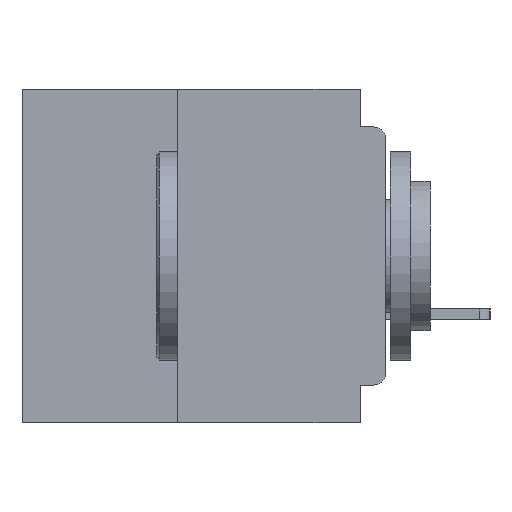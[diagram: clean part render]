
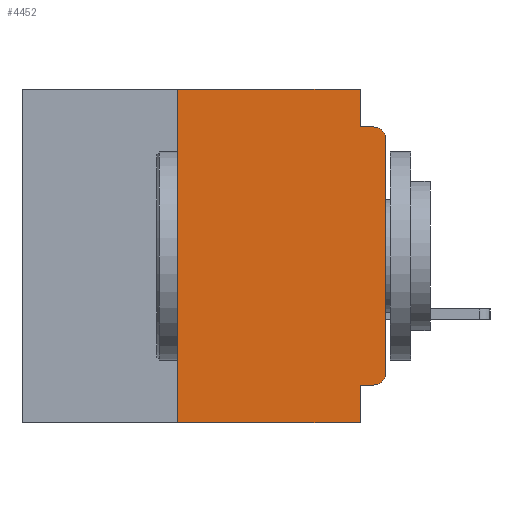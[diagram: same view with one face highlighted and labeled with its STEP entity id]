
A CAD part, left-side view. The second image highlights one B-rep face of the part: STEP entity #4452.
In plain terms, the highlighted planar face has unit normal (-1, 0, 0).
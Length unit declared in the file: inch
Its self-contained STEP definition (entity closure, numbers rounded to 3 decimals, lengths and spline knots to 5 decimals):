
#224 = LINE ( 'NONE', #22350, #27038 ) ;
#269 = EDGE_CURVE ( 'NONE', #44445, #28479, #2265, .T. ) ;
#1649 = EDGE_CURVE ( 'NONE', #26381, #44512, #7713, .T. ) ;
#1786 = AXIS2_PLACEMENT_3D ( 'NONE', #3555, #2990, #2940 ) ;
#1820 = VERTEX_POINT ( 'NONE', #19392 ) ;
#2265 = LINE ( 'NONE', #32004, #29104 ) ;
#2416 = VERTEX_POINT ( 'NONE', #4908 ) ;
#2940 = DIRECTION ( 'NONE',  ( 0., 0., -1. ) ) ;
#2990 = DIRECTION ( 'NONE',  ( 1., 0., 0. ) ) ;
#3138 = PLANE ( 'NONE',  #1786 ) ;
#3555 = CARTESIAN_POINT ( 'NONE',  ( 0., 0.437, 0. ) ) ;
#4447 = CIRCLE ( 'NONE', #4671, 0.015 ) ;
#4452 = ADVANCED_FACE ( 'NONE', ( #10829 ), #3138, .F. ) ;
#4671 = AXIS2_PLACEMENT_3D ( 'NONE', #34723, #13765, #38203 ) ;
#4908 = CARTESIAN_POINT ( 'NONE',  ( 0., 0.031, -0.045 ) ) ;
#4934 = VERTEX_POINT ( 'NONE', #20865 ) ;
#5201 = CIRCLE ( 'NONE', #21143, 0.015 ) ;
#5865 = LINE ( 'NONE', #12156, #14056 ) ;
#7415 = CARTESIAN_POINT ( 'NONE',  ( 0., 0.437, 0. ) ) ;
#7713 = LINE ( 'NONE', #23816, #26300 ) ;
#7797 = ORIENTED_EDGE ( 'NONE', *, *, #37757, .T. ) ;
#8063 = CARTESIAN_POINT ( 'NONE',  ( 0., 0.015, -0.06 ) ) ;
#8681 = ORIENTED_EDGE ( 'NONE', *, *, #1649, .F. ) ;
#10325 = CARTESIAN_POINT ( 'NONE',  ( 0., 0.031, 0. ) ) ;
#10829 = FACE_OUTER_BOUND ( 'NONE', #17352, .T. ) ;
#10909 = DIRECTION ( 'NONE',  ( 0., -1., 0. ) ) ;
#10977 = CARTESIAN_POINT ( 'NONE',  ( 0., 0., -0.045 ) ) ;
#11052 = EDGE_CURVE ( 'NONE', #34389, #2416, #5865, .T. ) ;
#11077 = ORIENTED_EDGE ( 'NONE', *, *, #31630, .T. ) ;
#11319 = ORIENTED_EDGE ( 'NONE', *, *, #22314, .T. ) ;
#11426 = CARTESIAN_POINT ( 'NONE',  ( 0., 0.015, -0.045 ) ) ;
#11463 = EDGE_CURVE ( 'NONE', #44512, #34389, #32624, .T. ) ;
#11566 = DIRECTION ( 'NONE',  ( 0., 0., -1. ) ) ;
#11826 = VECTOR ( 'NONE', #21428, 39.37008 ) ;
#12156 = CARTESIAN_POINT ( 'NONE',  ( 0., 0.031, 0. ) ) ;
#13763 = CARTESIAN_POINT ( 'NONE',  ( 0., 0.437, -0.4 ) ) ;
#13765 = DIRECTION ( 'NONE',  ( -1., 0., 0. ) ) ;
#14056 = VECTOR ( 'NONE', #40115, 39.37008 ) ;
#14590 = ORIENTED_EDGE ( 'NONE', *, *, #269, .F. ) ;
#16676 = EDGE_CURVE ( 'NONE', #2416, #35874, #30441, .T. ) ;
#17352 = EDGE_LOOP ( 'NONE', ( #7797, #11077, #20980, #42593, #22431, #8681, #31587, #39763, #14590, #11319 ) ) ;
#17910 = CARTESIAN_POINT ( 'NONE',  ( 0., 0.25, 0. ) ) ;
#19392 = CARTESIAN_POINT ( 'NONE',  ( 0., 0., -0.06 ) ) ;
#20865 = CARTESIAN_POINT ( 'NONE',  ( 0., 0.031, -0.4 ) ) ;
#20980 = ORIENTED_EDGE ( 'NONE', *, *, #16676, .F. ) ;
#21023 = CARTESIAN_POINT ( 'NONE',  ( 0., 0.015, -0.355 ) ) ;
#21143 = AXIS2_PLACEMENT_3D ( 'NONE', #8063, #32520, #11566 ) ;
#21428 = DIRECTION ( 'NONE',  ( 0., -1., 0. ) ) ;
#22265 = CARTESIAN_POINT ( 'NONE',  ( 0., 0.25, -0.4 ) ) ;
#22314 = EDGE_CURVE ( 'NONE', #44445, #32727, #4447, .T. ) ;
#22350 = CARTESIAN_POINT ( 'NONE',  ( 0., 0.031, -0.4 ) ) ;
#22431 = ORIENTED_EDGE ( 'NONE', *, *, #11463, .F. ) ;
#23705 = DIRECTION ( 'NONE',  ( 0., 0., 1. ) ) ;
#23816 = CARTESIAN_POINT ( 'NONE',  ( 0., 0.25, -0.4 ) ) ;
#26267 = CARTESIAN_POINT ( 'NONE',  ( 0., 0., 0. ) ) ;
#26300 = VECTOR ( 'NONE', #23705, 39.37008 ) ;
#26381 = VERTEX_POINT ( 'NONE', #22265 ) ;
#27038 = VECTOR ( 'NONE', #36353, 39.37008 ) ;
#28479 = VERTEX_POINT ( 'NONE', #34194 ) ;
#29104 = VECTOR ( 'NONE', #32100, 39.37008 ) ;
#29774 = DIRECTION ( 'NONE',  ( 0., 0., 1. ) ) ;
#30441 = LINE ( 'NONE', #10977, #11826 ) ;
#31587 = ORIENTED_EDGE ( 'NONE', *, *, #42357, .T. ) ;
#31630 = EDGE_CURVE ( 'NONE', #1820, #35874, #5201, .T. ) ;
#32004 = CARTESIAN_POINT ( 'NONE',  ( 0., 0., -0.355 ) ) ;
#32100 = DIRECTION ( 'NONE',  ( 0., 1., 0. ) ) ;
#32520 = DIRECTION ( 'NONE',  ( -1., 0., 0. ) ) ;
#32624 = LINE ( 'NONE', #7415, #40785 ) ;
#32727 = VERTEX_POINT ( 'NONE', #35012 ) ;
#34062 = VECTOR ( 'NONE', #41704, 39.37008 ) ;
#34194 = CARTESIAN_POINT ( 'NONE',  ( 0., 0.031, -0.355 ) ) ;
#34389 = VERTEX_POINT ( 'NONE', #10325 ) ;
#34723 = CARTESIAN_POINT ( 'NONE',  ( 0., 0.015, -0.34 ) ) ;
#35012 = CARTESIAN_POINT ( 'NONE',  ( 0., 0., -0.34 ) ) ;
#35874 = VERTEX_POINT ( 'NONE', #11426 ) ;
#36353 = DIRECTION ( 'NONE',  ( 0., 0., -1. ) ) ;
#37670 = EDGE_CURVE ( 'NONE', #28479, #4934, #224, .T. ) ;
#37757 = EDGE_CURVE ( 'NONE', #32727, #1820, #42314, .T. ) ;
#38203 = DIRECTION ( 'NONE',  ( 0., 0., -1. ) ) ;
#39763 = ORIENTED_EDGE ( 'NONE', *, *, #37670, .F. ) ;
#40115 = DIRECTION ( 'NONE',  ( 0., 0., -1. ) ) ;
#40785 = VECTOR ( 'NONE', #10909, 39.37008 ) ;
#41207 = VECTOR ( 'NONE', #29774, 39.37008 ) ;
#41704 = DIRECTION ( 'NONE',  ( 0., -1., 0. ) ) ;
#42314 = LINE ( 'NONE', #26267, #41207 ) ;
#42357 = EDGE_CURVE ( 'NONE', #26381, #4934, #43309, .T. ) ;
#42593 = ORIENTED_EDGE ( 'NONE', *, *, #11052, .F. ) ;
#43309 = LINE ( 'NONE', #13763, #34062 ) ;
#44445 = VERTEX_POINT ( 'NONE', #21023 ) ;
#44512 = VERTEX_POINT ( 'NONE', #17910 ) ;
